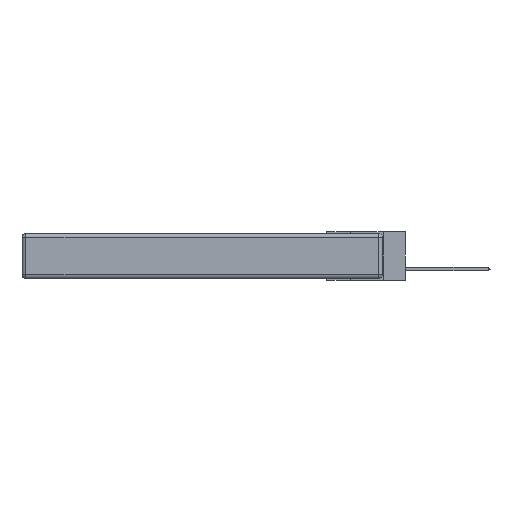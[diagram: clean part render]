
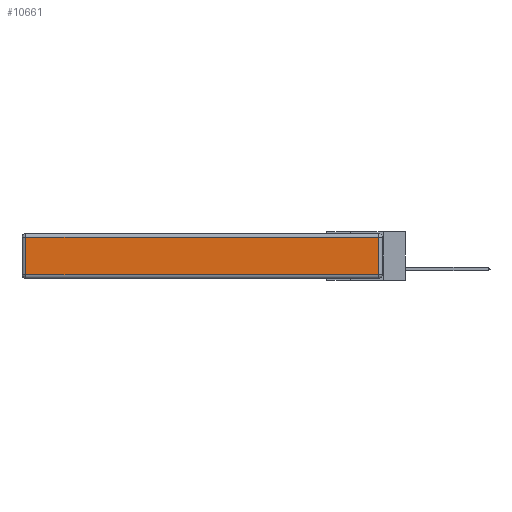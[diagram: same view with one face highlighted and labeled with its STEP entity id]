
A CAD part, left-side view. The second image highlights one B-rep face of the part: STEP entity #10661.
In plain terms, the highlighted planar face has unit normal (-1, 0, 0).
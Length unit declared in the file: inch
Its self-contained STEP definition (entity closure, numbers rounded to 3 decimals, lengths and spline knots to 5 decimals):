
#96 = VECTOR ( 'NONE', #1761, 39.37008 ) ;
#457 = CARTESIAN_POINT ( 'NONE',  ( 0., 2.75, -0.03 ) ) ;
#1539 = DIRECTION ( 'NONE',  ( -1., 0., 0. ) ) ;
#1761 = DIRECTION ( 'NONE',  ( 0., 0., 1. ) ) ;
#2866 = DIRECTION ( 'NONE',  ( 0., -1., 0. ) ) ;
#2867 = ORIENTED_EDGE ( 'NONE', *, *, #13203, .T. ) ;
#3586 = ORIENTED_EDGE ( 'NONE', *, *, #3940, .T. ) ;
#3750 = ORIENTED_EDGE ( 'NONE', *, *, #13034, .T. ) ;
#3940 = EDGE_CURVE ( 'NONE', #13907, #13159, #14402, .T. ) ;
#4562 = CARTESIAN_POINT ( 'NONE',  ( 0., 2.72, -0.313 ) ) ;
#5188 = CARTESIAN_POINT ( 'NONE',  ( 0., 0., -0.313 ) ) ;
#6010 = VECTOR ( 'NONE', #2866, 39.37008 ) ;
#6161 = CARTESIAN_POINT ( 'NONE',  ( 0., 0.03, -0.343 ) ) ;
#6221 = VERTEX_POINT ( 'NONE', #10555 ) ;
#6956 = CARTESIAN_POINT ( 'NONE',  ( 0., 2.72, -0.343 ) ) ;
#7115 = DIRECTION ( 'NONE',  ( 0., 0., -1. ) ) ;
#7395 = CARTESIAN_POINT ( 'NONE',  ( 0., 0.03, -0.313 ) ) ;
#8261 = VECTOR ( 'NONE', #13861, 39.37008 ) ;
#8294 = PLANE ( 'NONE',  #12080 ) ;
#8340 = CARTESIAN_POINT ( 'NONE',  ( 0., 0., -0.343 ) ) ;
#8586 = VERTEX_POINT ( 'NONE', #9639 ) ;
#8977 = EDGE_CURVE ( 'NONE', #8586, #6221, #10858, .T. ) ;
#9207 = DIRECTION ( 'NONE',  ( 0., 0., 1. ) ) ;
#9639 = CARTESIAN_POINT ( 'NONE',  ( 0., 0.03, -0.03 ) ) ;
#10056 = ORIENTED_EDGE ( 'NONE', *, *, #8977, .T. ) ;
#10555 = CARTESIAN_POINT ( 'NONE',  ( 0., 2.72, -0.03 ) ) ;
#10661 = ADVANCED_FACE ( 'NONE', ( #11517 ), #8294, .T. ) ;
#10858 = LINE ( 'NONE', #457, #8261 ) ;
#10935 = VECTOR ( 'NONE', #7115, 39.37008 ) ;
#11517 = FACE_OUTER_BOUND ( 'NONE', #14407, .T. ) ;
#11990 = LINE ( 'NONE', #6956, #10935 ) ;
#12080 = AXIS2_PLACEMENT_3D ( 'NONE', #8340, #1539, #9207 ) ;
#13034 = EDGE_CURVE ( 'NONE', #6221, #13907, #11990, .T. ) ;
#13159 = VERTEX_POINT ( 'NONE', #7395 ) ;
#13203 = EDGE_CURVE ( 'NONE', #13159, #8586, #13929, .T. ) ;
#13861 = DIRECTION ( 'NONE',  ( 0., 1., 0. ) ) ;
#13907 = VERTEX_POINT ( 'NONE', #4562 ) ;
#13929 = LINE ( 'NONE', #6161, #96 ) ;
#14402 = LINE ( 'NONE', #5188, #6010 ) ;
#14407 = EDGE_LOOP ( 'NONE', ( #3586, #2867, #10056, #3750 ) ) ;
